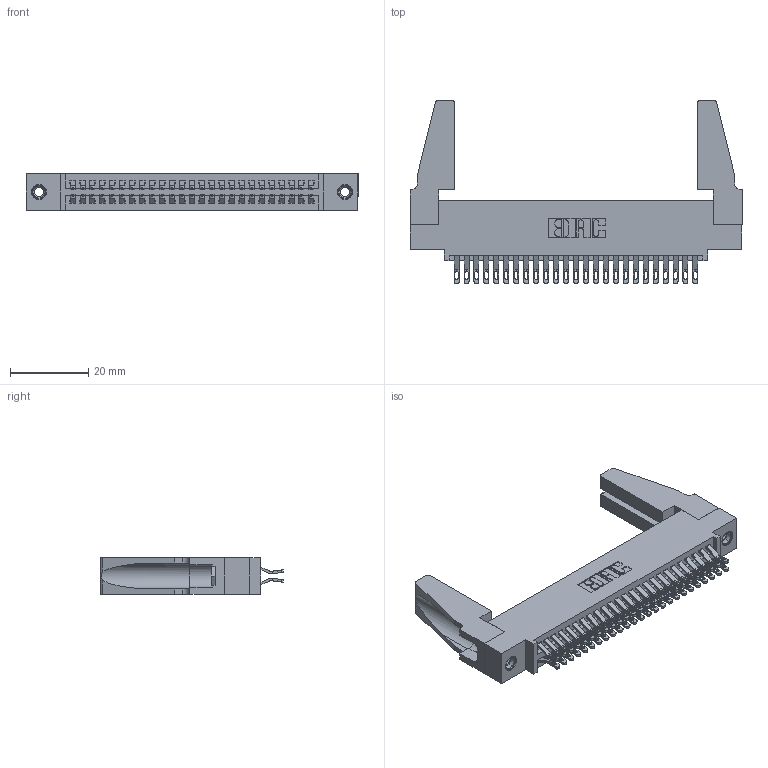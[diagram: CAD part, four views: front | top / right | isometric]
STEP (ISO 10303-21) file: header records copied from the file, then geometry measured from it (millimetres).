
FILE_DESCRIPTION (( 'STEP AP203' ), '1' );
FILE_NAME ('395-050-555-588.STEP', '2019-10-19T13:57:44', ( '' ), ( '' ), 'SwSTEP 2.0', 'SolidWorks 2016', '' );
FILE_SCHEMA (( 'CONFIG_CONTROL_DESIGN' ));
Length unit declared in the file: inch
Products named in the file (5): 345 Part_0.110 Offset - 0.156 Dia-TH; 345-292-001_555 Tail; 345-250-001_345-250-001-102; 345-220-078_345-220-088; 395-050-555-588
Assembly tree (55 placements, depth 2):
  395-050-555-588
    345 Part_0.110 Offset - 0.156 Dia-TH
    345-292-001_555 Tail  x50
    345-250-001_345-250-001-102  x2
    345-220-078_345-220-088  x2
Bounding box: 84.73 x 46.79 x 9.4 mm (x, y, z)
Volume: 11397.5 mm3; surface area: 15429.9 mm2
Topology: 55 solids, 55 shells, 3054 faces, 9517 edges, 6334 vertices
Faces by surface type: plane 1706, cylinder 1332, cone 12, torus 4
Entity records: 24510 total; most frequent: CARTESIAN_POINT 4156, ORIENTED_EDGE 4020, DIRECTION 3658, EDGE_CURVE 2010, LINE 1716, VECTOR 1716, VERTEX_POINT 1334, AXIS2_PLACEMENT_3D 971
